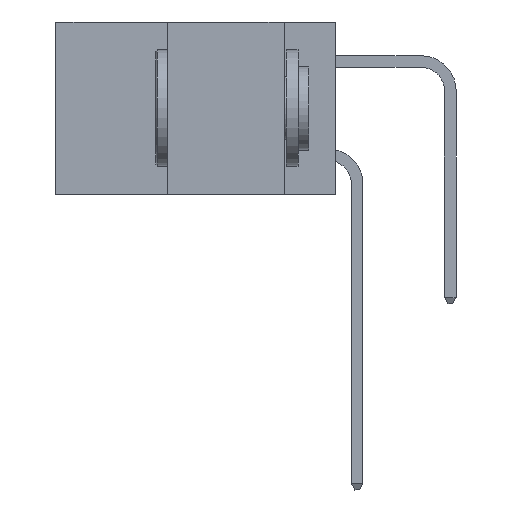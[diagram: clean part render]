
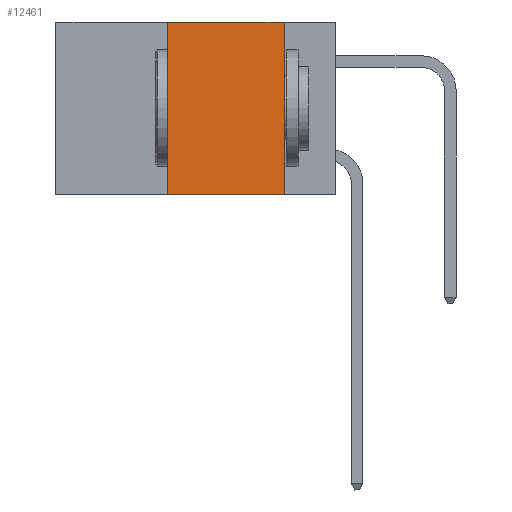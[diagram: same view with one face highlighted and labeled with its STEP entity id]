
A CAD part, left-side view. The second image highlights one B-rep face of the part: STEP entity #12461.
In plain terms, the highlighted planar face has unit normal (-1, 0, 0).
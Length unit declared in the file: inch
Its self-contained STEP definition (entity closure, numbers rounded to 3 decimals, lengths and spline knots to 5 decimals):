
#230 = CARTESIAN_POINT ( 'NONE',  ( 0., 0.36, -0.37 ) ) ;
#339 = VERTEX_POINT ( 'NONE', #6341 ) ;
#1307 = VERTEX_POINT ( 'NONE', #14768 ) ;
#1501 = EDGE_CURVE ( 'NONE', #1307, #3086, #3181, .T. ) ;
#2212 = DIRECTION ( 'NONE',  ( 0., 0., 1. ) ) ;
#2531 = DIRECTION ( 'NONE',  ( 0., -1., 0. ) ) ;
#2737 = CARTESIAN_POINT ( 'NONE',  ( 0., 0.6, 0. ) ) ;
#3049 = FACE_OUTER_BOUND ( 'NONE', #15472, .T. ) ;
#3086 = VERTEX_POINT ( 'NONE', #15917 ) ;
#3181 = LINE ( 'NONE', #23310, #22785 ) ;
#4829 = CARTESIAN_POINT ( 'NONE',  ( 0., 0.6, -0.37 ) ) ;
#4846 = VERTEX_POINT ( 'NONE', #230 ) ;
#4949 = EDGE_CURVE ( 'NONE', #339, #1307, #15904, .T. ) ;
#5410 = AXIS2_PLACEMENT_3D ( 'NONE', #2737, #24225, #14410 ) ;
#6341 = CARTESIAN_POINT ( 'NONE',  ( 0., 0.36, 0. ) ) ;
#6491 = ORIENTED_EDGE ( 'NONE', *, *, #16464, .F. ) ;
#8328 = PLANE ( 'NONE',  #5410 ) ;
#8694 = VECTOR ( 'NONE', #14587, 39.37008 ) ;
#9281 = VECTOR ( 'NONE', #2531, 39.37008 ) ;
#9315 = ORIENTED_EDGE ( 'NONE', *, *, #12496, .T. ) ;
#9949 = ORIENTED_EDGE ( 'NONE', *, *, #4949, .F. ) ;
#11191 = VECTOR ( 'NONE', #2212, 39.37008 ) ;
#12337 = LINE ( 'NONE', #4829, #8694 ) ;
#12461 = ADVANCED_FACE ( 'NONE', ( #3049 ), #8328, .F. ) ;
#12496 = EDGE_CURVE ( 'NONE', #4846, #3086, #12337, .T. ) ;
#14410 = DIRECTION ( 'NONE',  ( 0., 0., -1. ) ) ;
#14587 = DIRECTION ( 'NONE',  ( 0., -1., 0. ) ) ;
#14768 = CARTESIAN_POINT ( 'NONE',  ( 0., 0.11, 0. ) ) ;
#15472 = EDGE_LOOP ( 'NONE', ( #24453, #9949, #6491, #9315 ) ) ;
#15904 = LINE ( 'NONE', #21945, #9281 ) ;
#15917 = CARTESIAN_POINT ( 'NONE',  ( 0., 0.11, -0.37 ) ) ;
#16464 = EDGE_CURVE ( 'NONE', #4846, #339, #22105, .T. ) ;
#19596 = CARTESIAN_POINT ( 'NONE',  ( 0., 0.36, 0. ) ) ;
#21637 = DIRECTION ( 'NONE',  ( 0., 0., -1. ) ) ;
#21945 = CARTESIAN_POINT ( 'NONE',  ( 0., 0.6, 0. ) ) ;
#22105 = LINE ( 'NONE', #19596, #11191 ) ;
#22785 = VECTOR ( 'NONE', #21637, 39.37008 ) ;
#23310 = CARTESIAN_POINT ( 'NONE',  ( 0., 0.11, 0. ) ) ;
#24225 = DIRECTION ( 'NONE',  ( 1., 0., 0. ) ) ;
#24453 = ORIENTED_EDGE ( 'NONE', *, *, #1501, .F. ) ;
